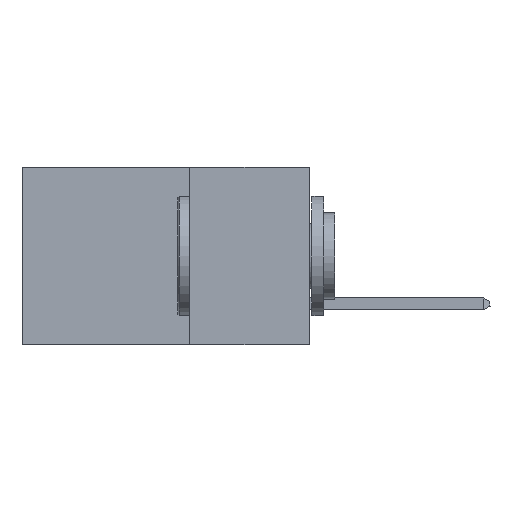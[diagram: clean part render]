
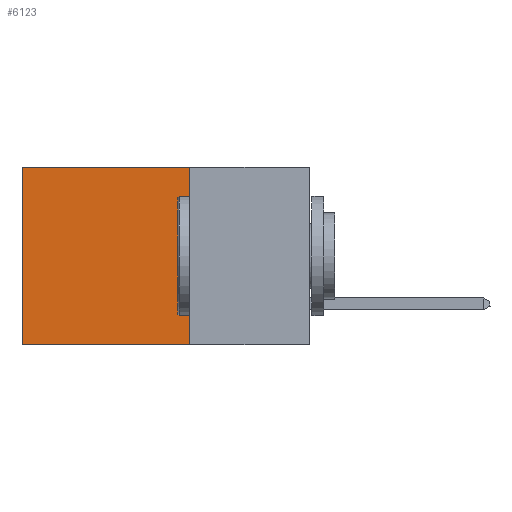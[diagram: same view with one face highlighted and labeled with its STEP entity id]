
A CAD part, left-side view. The second image highlights one B-rep face of the part: STEP entity #6123.
In plain terms, the highlighted planar face has unit normal (-1, 0, 0).
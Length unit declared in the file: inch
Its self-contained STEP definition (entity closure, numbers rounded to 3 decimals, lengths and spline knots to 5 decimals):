
#1384 = DIRECTION ( 'NONE',  ( 0., 0., -1. ) ) ;
#3924 = ORIENTED_EDGE ( 'NONE', *, *, #36239, .F. ) ;
#4526 = VECTOR ( 'NONE', #17928, 39.37008 ) ;
#6123 = ADVANCED_FACE ( 'NONE', ( #10375 ), #17578, .F. ) ;
#6658 = VECTOR ( 'NONE', #23027, 39.37008 ) ;
#6792 = DIRECTION ( 'NONE',  ( 0., 1., 0. ) ) ;
#7979 = CARTESIAN_POINT ( 'NONE',  ( 0.2875, 0.25, -0.37 ) ) ;
#9218 = AXIS2_PLACEMENT_3D ( 'NONE', #39790, #20808, #1384 ) ;
#9478 = ORIENTED_EDGE ( 'NONE', *, *, #36426, .F. ) ;
#9734 = EDGE_LOOP ( 'NONE', ( #36235, #3924, #9478, #35090 ) ) ;
#10375 = FACE_OUTER_BOUND ( 'NONE', #9734, .T. ) ;
#14559 = CARTESIAN_POINT ( 'NONE',  ( 0.2875, 0.6, 0. ) ) ;
#14672 = VECTOR ( 'NONE', #6792, 39.37008 ) ;
#14785 = VECTOR ( 'NONE', #34888, 39.37008 ) ;
#15409 = CARTESIAN_POINT ( 'NONE',  ( 0.2875, 0.25, 0. ) ) ;
#15482 = EDGE_CURVE ( 'NONE', #29636, #17090, #30194, .T. ) ;
#15618 = VERTEX_POINT ( 'NONE', #15409 ) ;
#15804 = LINE ( 'NONE', #41014, #14785 ) ;
#17090 = VERTEX_POINT ( 'NONE', #31215 ) ;
#17578 = PLANE ( 'NONE',  #9218 ) ;
#17928 = DIRECTION ( 'NONE',  ( 0., 0., -1. ) ) ;
#18218 = VERTEX_POINT ( 'NONE', #7979 ) ;
#20808 = DIRECTION ( 'NONE',  ( 1., 0., 0. ) ) ;
#23027 = DIRECTION ( 'NONE',  ( 0., 0., -1. ) ) ;
#23193 = LINE ( 'NONE', #35530, #14672 ) ;
#23792 = LINE ( 'NONE', #38820, #6658 ) ;
#29636 = VERTEX_POINT ( 'NONE', #14559 ) ;
#30194 = LINE ( 'NONE', #33863, #4526 ) ;
#31215 = CARTESIAN_POINT ( 'NONE',  ( 0.2875, 0.6, -0.37 ) ) ;
#33863 = CARTESIAN_POINT ( 'NONE',  ( 0.2875, 0.6, 0. ) ) ;
#34888 = DIRECTION ( 'NONE',  ( 0., 1., 0. ) ) ;
#35090 = ORIENTED_EDGE ( 'NONE', *, *, #37488, .T. ) ;
#35530 = CARTESIAN_POINT ( 'NONE',  ( 0.2875, 0.25, 0. ) ) ;
#36235 = ORIENTED_EDGE ( 'NONE', *, *, #15482, .T. ) ;
#36239 = EDGE_CURVE ( 'NONE', #18218, #17090, #15804, .T. ) ;
#36426 = EDGE_CURVE ( 'NONE', #15618, #18218, #23792, .T. ) ;
#37488 = EDGE_CURVE ( 'NONE', #15618, #29636, #23193, .T. ) ;
#38820 = CARTESIAN_POINT ( 'NONE',  ( 0.2875, 0.25, 0. ) ) ;
#39790 = CARTESIAN_POINT ( 'NONE',  ( 0.2875, 0.25, 0. ) ) ;
#41014 = CARTESIAN_POINT ( 'NONE',  ( 0.2875, 0.25, -0.37 ) ) ;
